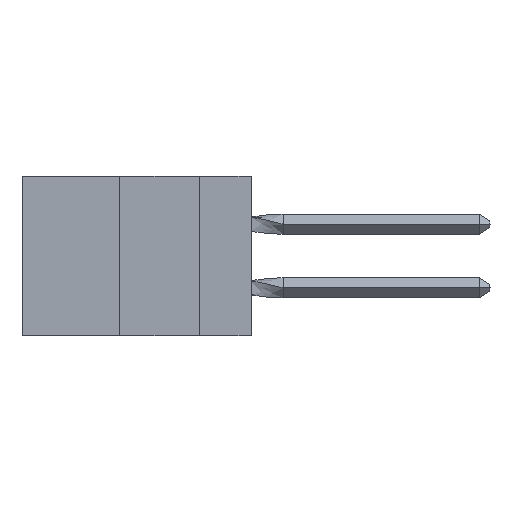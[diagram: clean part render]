
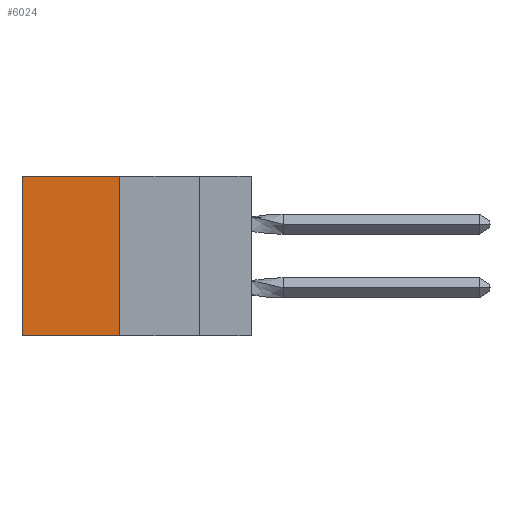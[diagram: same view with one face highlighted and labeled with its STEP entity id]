
A CAD part, left-side view. The second image highlights one B-rep face of the part: STEP entity #6024.
In plain terms, the highlighted planar face has unit normal (-1, 0, 0).
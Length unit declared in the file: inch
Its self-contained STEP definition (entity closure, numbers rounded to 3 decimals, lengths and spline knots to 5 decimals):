
#496 = LINE ( 'NONE', #10073, #15705 ) ;
#1057 = VERTEX_POINT ( 'NONE', #13003 ) ;
#2481 = CARTESIAN_POINT ( 'NONE',  ( 0.305, 0.413, 0. ) ) ;
#2506 = VECTOR ( 'NONE', #17539, 39.37008 ) ;
#3300 = EDGE_CURVE ( 'NONE', #4514, #8391, #10827, .T. ) ;
#4514 = VERTEX_POINT ( 'NONE', #18636 ) ;
#6024 = ADVANCED_FACE ( 'NONE', ( #15574 ), #12726, .F. ) ;
#6409 = VECTOR ( 'NONE', #17795, 39.37008 ) ;
#6941 = ORIENTED_EDGE ( 'NONE', *, *, #13468, .T. ) ;
#7660 = EDGE_CURVE ( 'NONE', #1057, #8391, #11921, .T. ) ;
#8320 = VERTEX_POINT ( 'NONE', #2481 ) ;
#8391 = VERTEX_POINT ( 'NONE', #11256 ) ;
#8566 = DIRECTION ( 'NONE',  ( 1., 0., 0. ) ) ;
#9673 = AXIS2_PLACEMENT_3D ( 'NONE', #15815, #8566, #9852 ) ;
#9852 = DIRECTION ( 'NONE',  ( 0., 0., -1. ) ) ;
#10073 = CARTESIAN_POINT ( 'NONE',  ( 0.305, 0.413, 0. ) ) ;
#10827 = LINE ( 'NONE', #17746, #2506 ) ;
#11256 = CARTESIAN_POINT ( 'NONE',  ( 0.305, 0.72, -0.5 ) ) ;
#11618 = ORIENTED_EDGE ( 'NONE', *, *, #3300, .F. ) ;
#11921 = LINE ( 'NONE', #19083, #6409 ) ;
#12066 = VECTOR ( 'NONE', #15749, 39.37008 ) ;
#12232 = EDGE_CURVE ( 'NONE', #8320, #4514, #18109, .T. ) ;
#12726 = PLANE ( 'NONE',  #9673 ) ;
#13003 = CARTESIAN_POINT ( 'NONE',  ( 0.305, 0.72, 0. ) ) ;
#13148 = ORIENTED_EDGE ( 'NONE', *, *, #7660, .T. ) ;
#13468 = EDGE_CURVE ( 'NONE', #8320, #1057, #496, .T. ) ;
#14288 = ORIENTED_EDGE ( 'NONE', *, *, #12232, .F. ) ;
#14500 = DIRECTION ( 'NONE',  ( 0., 1., 0. ) ) ;
#14621 = EDGE_LOOP ( 'NONE', ( #13148, #11618, #14288, #6941 ) ) ;
#15574 = FACE_OUTER_BOUND ( 'NONE', #14621, .T. ) ;
#15705 = VECTOR ( 'NONE', #14500, 39.37008 ) ;
#15749 = DIRECTION ( 'NONE',  ( 0., 0., -1. ) ) ;
#15815 = CARTESIAN_POINT ( 'NONE',  ( 0.305, 0.413, -0.5 ) ) ;
#17208 = CARTESIAN_POINT ( 'NONE',  ( 0.305, 0.413, -0.5 ) ) ;
#17539 = DIRECTION ( 'NONE',  ( 0., 1., 0. ) ) ;
#17746 = CARTESIAN_POINT ( 'NONE',  ( 0.305, 0.413, -0.5 ) ) ;
#17795 = DIRECTION ( 'NONE',  ( 0., 0., -1. ) ) ;
#18109 = LINE ( 'NONE', #17208, #12066 ) ;
#18636 = CARTESIAN_POINT ( 'NONE',  ( 0.305, 0.413, -0.5 ) ) ;
#19083 = CARTESIAN_POINT ( 'NONE',  ( 0.305, 0.72, -0.5 ) ) ;
